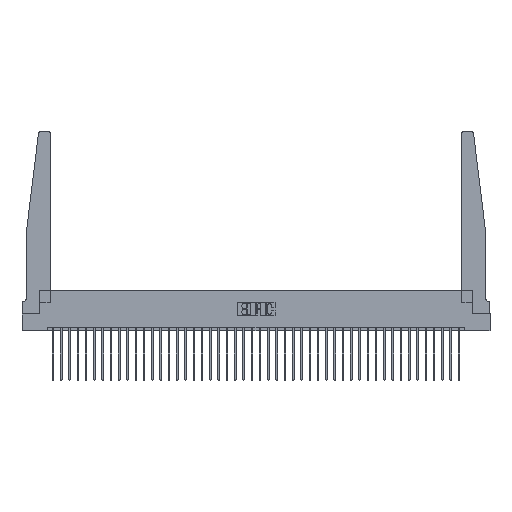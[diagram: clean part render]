
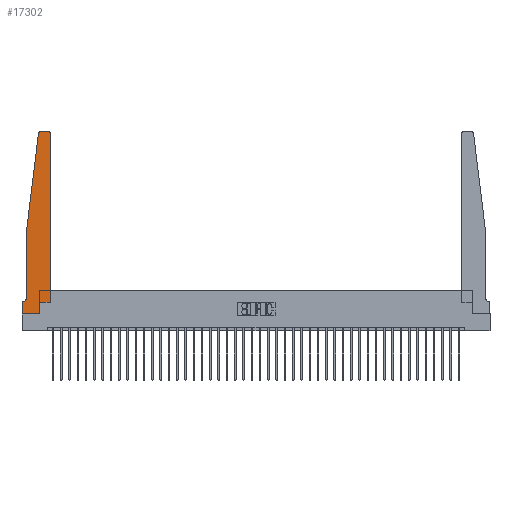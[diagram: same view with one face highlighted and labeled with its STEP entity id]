
A CAD part, top view. The second image highlights one B-rep face of the part: STEP entity #17302.
In plain terms, the highlighted planar face has unit normal (0, 0, 1).
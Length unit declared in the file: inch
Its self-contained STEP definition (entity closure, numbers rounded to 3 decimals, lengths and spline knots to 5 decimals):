
#117 = CARTESIAN_POINT ( 'NONE',  ( 0., 0., 0.37 ) ) ;
#197 = EDGE_CURVE ( 'NONE', #21042, #25213, #22646, .T. ) ;
#257 = VERTEX_POINT ( 'NONE', #19673 ) ;
#771 = VECTOR ( 'NONE', #18883, 39.37008 ) ;
#892 = ORIENTED_EDGE ( 'NONE', *, *, #30483, .T. ) ;
#1230 = LINE ( 'NONE', #23883, #771 ) ;
#1376 = CARTESIAN_POINT ( 'NONE',  ( 0.2605, 0.18, 0.37 ) ) ;
#1556 = VERTEX_POINT ( 'NONE', #24421 ) ;
#1682 = EDGE_CURVE ( 'NONE', #30028, #34232, #13854, .T. ) ;
#2011 = VECTOR ( 'NONE', #22776, 39.37008 ) ;
#2449 = CARTESIAN_POINT ( 'NONE',  ( 0.25, 2.75, 0.37 ) ) ;
#3126 = CIRCLE ( 'NONE', #31661, 0.03 ) ;
#3449 = ORIENTED_EDGE ( 'NONE', *, *, #19756, .T. ) ;
#3689 = EDGE_LOOP ( 'NONE', ( #24056, #33244, #31141, #28715, #25956, #17352, #3449, #3941, #19415, #5447, #23162, #892 ) ) ;
#3941 = ORIENTED_EDGE ( 'NONE', *, *, #18477, .T. ) ;
#4037 = CIRCLE ( 'NONE', #5484, 0.03 ) ;
#4246 = CARTESIAN_POINT ( 'NONE',  ( 0.065, 1.25, 0.37 ) ) ;
#4271 = VERTEX_POINT ( 'NONE', #7688 ) ;
#4293 = EDGE_CURVE ( 'NONE', #24578, #14932, #22838, .T. ) ;
#5447 = ORIENTED_EDGE ( 'NONE', *, *, #19902, .T. ) ;
#5484 = AXIS2_PLACEMENT_3D ( 'NONE', #12932, #7136, #10213 ) ;
#6120 = VECTOR ( 'NONE', #22481, 39.37008 ) ;
#7136 = DIRECTION ( 'NONE',  ( 0., 0., 1. ) ) ;
#7231 = DIRECTION ( 'NONE',  ( -1., 0., 0. ) ) ;
#7396 = LINE ( 'NONE', #30792, #35057 ) ;
#7480 = CIRCLE ( 'NONE', #23757, 0.05 ) ;
#7688 = CARTESIAN_POINT ( 'NONE',  ( 0.065, 0.2375, 0.37 ) ) ;
#7918 = VECTOR ( 'NONE', #10568, 39.37008 ) ;
#8153 = CARTESIAN_POINT ( 'NONE',  ( 0.425, 2.72, 0.37 ) ) ;
#8504 = CARTESIAN_POINT ( 'NONE',  ( 0.015, 0.1875, 0.37 ) ) ;
#8592 = DIRECTION ( 'NONE',  ( 0., -1., 0. ) ) ;
#8753 = EDGE_CURVE ( 'NONE', #257, #25712, #20195, .T. ) ;
#8787 = EDGE_CURVE ( 'NONE', #4271, #21042, #7480, .T. ) ;
#8800 = EDGE_CURVE ( 'NONE', #14932, #4271, #35172, .T. ) ;
#8892 = LINE ( 'NONE', #117, #23776 ) ;
#9509 = CARTESIAN_POINT ( 'NONE',  ( 0.065, 1.25, 0.37 ) ) ;
#9693 = DIRECTION ( 'NONE',  ( 0., 0., -1. ) ) ;
#10213 = DIRECTION ( 'NONE',  ( 1., 0., 0. ) ) ;
#10450 = DIRECTION ( 'NONE',  ( 0., 1., 0. ) ) ;
#10568 = DIRECTION ( 'NONE',  ( 0., -1., 0. ) ) ;
#10664 = FACE_OUTER_BOUND ( 'NONE', #3689, .T. ) ;
#11486 = CARTESIAN_POINT ( 'NONE',  ( 0.395, 2.72, 0.37 ) ) ;
#12531 = EDGE_CURVE ( 'NONE', #28299, #12841, #1230, .T. ) ;
#12841 = VERTEX_POINT ( 'NONE', #1376 ) ;
#12906 = CARTESIAN_POINT ( 'NONE',  ( 0.015, 0.2375, 0.37 ) ) ;
#12932 = CARTESIAN_POINT ( 'NONE',  ( 0.27653, 2.72, 0.37 ) ) ;
#13320 = AXIS2_PLACEMENT_3D ( 'NONE', #32453, #29908, #32696 ) ;
#13854 = LINE ( 'NONE', #21196, #36252 ) ;
#14932 = VERTEX_POINT ( 'NONE', #9509 ) ;
#16030 = CARTESIAN_POINT ( 'NONE',  ( 0., 0.1875, 0.37 ) ) ;
#17302 = ADVANCED_FACE ( 'NONE', ( #10664 ), #26812, .T. ) ;
#17352 = ORIENTED_EDGE ( 'NONE', *, *, #197, .T. ) ;
#18477 = EDGE_CURVE ( 'NONE', #1556, #28299, #7396, .T. ) ;
#18883 = DIRECTION ( 'NONE',  ( 0., 1., 0. ) ) ;
#18931 = VECTOR ( 'NONE', #32970, 39.37008 ) ;
#19415 = ORIENTED_EDGE ( 'NONE', *, *, #12531, .T. ) ;
#19673 = CARTESIAN_POINT ( 'NONE',  ( 0.395, 2.75, 0.37 ) ) ;
#19756 = EDGE_CURVE ( 'NONE', #25213, #1556, #8892, .T. ) ;
#19902 = EDGE_CURVE ( 'NONE', #12841, #30028, #35697, .T. ) ;
#20195 = LINE ( 'NONE', #2449, #6120 ) ;
#21042 = VERTEX_POINT ( 'NONE', #8504 ) ;
#21196 = CARTESIAN_POINT ( 'NONE',  ( 0.425, 0.18, 0.37 ) ) ;
#21314 = CARTESIAN_POINT ( 'NONE',  ( 0.2605, 0., 0.37 ) ) ;
#22481 = DIRECTION ( 'NONE',  ( -1., 0., 0. ) ) ;
#22646 = LINE ( 'NONE', #28360, #2011 ) ;
#22776 = DIRECTION ( 'NONE',  ( -1., 0., 0. ) ) ;
#22838 = LINE ( 'NONE', #24508, #18931 ) ;
#23162 = ORIENTED_EDGE ( 'NONE', *, *, #1682, .T. ) ;
#23757 = AXIS2_PLACEMENT_3D ( 'NONE', #12906, #9693, #7231 ) ;
#23776 = VECTOR ( 'NONE', #8592, 39.37008 ) ;
#23883 = CARTESIAN_POINT ( 'NONE',  ( 0.2605, 0.18, 0.37 ) ) ;
#24056 = ORIENTED_EDGE ( 'NONE', *, *, #8753, .T. ) ;
#24234 = CARTESIAN_POINT ( 'NONE',  ( 0.24675, 2.72367, 0.37 ) ) ;
#24421 = CARTESIAN_POINT ( 'NONE',  ( 0., 0., 0.37 ) ) ;
#24508 = CARTESIAN_POINT ( 'NONE',  ( 0.065, 1.25, 0.37 ) ) ;
#24578 = VERTEX_POINT ( 'NONE', #24234 ) ;
#25213 = VERTEX_POINT ( 'NONE', #16030 ) ;
#25332 = DIRECTION ( 'NONE',  ( 0., 0., 1. ) ) ;
#25584 = DIRECTION ( 'NONE',  ( 1., 0., 0. ) ) ;
#25712 = VERTEX_POINT ( 'NONE', #35223 ) ;
#25956 = ORIENTED_EDGE ( 'NONE', *, *, #8787, .T. ) ;
#26375 = CARTESIAN_POINT ( 'NONE',  ( 0.425, 0.18, 0.37 ) ) ;
#26812 = PLANE ( 'NONE',  #13320 ) ;
#28299 = VERTEX_POINT ( 'NONE', #21314 ) ;
#28360 = CARTESIAN_POINT ( 'NONE',  ( 0.065, 0.1875, 0.37 ) ) ;
#28715 = ORIENTED_EDGE ( 'NONE', *, *, #8800, .T. ) ;
#29458 = EDGE_CURVE ( 'NONE', #25712, #24578, #4037, .T. ) ;
#29533 = VECTOR ( 'NONE', #34240, 39.37008 ) ;
#29908 = DIRECTION ( 'NONE',  ( 0., 0., 1. ) ) ;
#30028 = VERTEX_POINT ( 'NONE', #26375 ) ;
#30483 = EDGE_CURVE ( 'NONE', #34232, #257, #3126, .T. ) ;
#30792 = CARTESIAN_POINT ( 'NONE',  ( 0., 0., 0.37 ) ) ;
#31141 = ORIENTED_EDGE ( 'NONE', *, *, #4293, .T. ) ;
#31661 = AXIS2_PLACEMENT_3D ( 'NONE', #11486, #25332, #25584 ) ;
#32453 = CARTESIAN_POINT ( 'NONE',  ( 0., 0.1875, 0.37 ) ) ;
#32696 = DIRECTION ( 'NONE',  ( 1., 0., 0. ) ) ;
#32970 = DIRECTION ( 'NONE',  ( -0.122, -0.992, 0. ) ) ;
#33244 = ORIENTED_EDGE ( 'NONE', *, *, #29458, .T. ) ;
#34122 = CARTESIAN_POINT ( 'NONE',  ( 0.425, 0.18, 0.37 ) ) ;
#34232 = VERTEX_POINT ( 'NONE', #8153 ) ;
#34240 = DIRECTION ( 'NONE',  ( 1., 0., 0. ) ) ;
#35057 = VECTOR ( 'NONE', #36078, 39.37008 ) ;
#35172 = LINE ( 'NONE', #4246, #7918 ) ;
#35223 = CARTESIAN_POINT ( 'NONE',  ( 0.27653, 2.75, 0.37 ) ) ;
#35697 = LINE ( 'NONE', #34122, #29533 ) ;
#36078 = DIRECTION ( 'NONE',  ( 1., 0., 0. ) ) ;
#36252 = VECTOR ( 'NONE', #10450, 39.37008 ) ;
